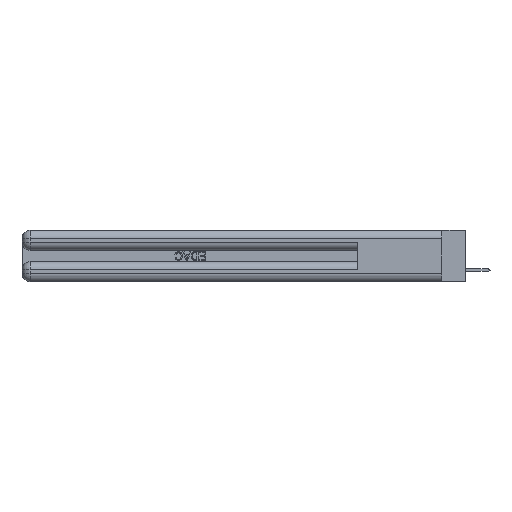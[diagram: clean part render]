
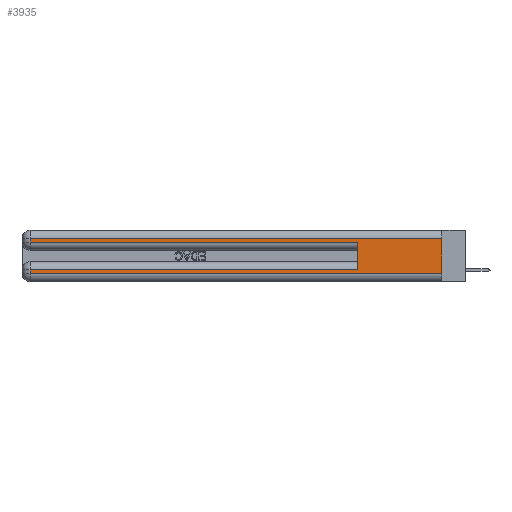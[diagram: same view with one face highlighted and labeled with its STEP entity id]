
A CAD part, left-side view. The second image highlights one B-rep face of the part: STEP entity #3935.
In plain terms, the highlighted planar face has unit normal (-1, 0, 0).
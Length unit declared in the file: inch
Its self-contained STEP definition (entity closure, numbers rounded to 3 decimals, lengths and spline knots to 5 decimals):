
#393 = ORIENTED_EDGE ( 'NONE', *, *, #5907, .F. ) ;
#418 = DIRECTION ( 'NONE',  ( 0., -1., 0. ) ) ;
#877 = VECTOR ( 'NONE', #418, 39.37008 ) ;
#1782 = ORIENTED_EDGE ( 'NONE', *, *, #13395, .T. ) ;
#3054 = DIRECTION ( 'NONE',  ( 0., 0., -1. ) ) ;
#3144 = EDGE_CURVE ( 'NONE', #14820, #27483, #23583, .T. ) ;
#3613 = VECTOR ( 'NONE', #27817, 39.37008 ) ;
#3715 = CARTESIAN_POINT ( 'NONE',  ( 0., 0., 0.31 ) ) ;
#3935 = ADVANCED_FACE ( 'NONE', ( #10803 ), #21529, .F. ) ;
#4452 = LINE ( 'NONE', #12826, #22128 ) ;
#4859 = CARTESIAN_POINT ( 'NONE',  ( 0., 0.6, 0.085 ) ) ;
#5136 = CARTESIAN_POINT ( 'NONE',  ( 0., 2.94, 0.37 ) ) ;
#5847 = EDGE_CURVE ( 'NONE', #24439, #14976, #4452, .T. ) ;
#5859 = LINE ( 'NONE', #25471, #12469 ) ;
#5907 = EDGE_CURVE ( 'NONE', #8286, #31642, #16191, .T. ) ;
#5970 = DIRECTION ( 'NONE',  ( 0., 1., 0. ) ) ;
#6474 = AXIS2_PLACEMENT_3D ( 'NONE', #27050, #18943, #21776 ) ;
#8118 = CARTESIAN_POINT ( 'NONE',  ( 0., 0., 0.085 ) ) ;
#8179 = EDGE_CURVE ( 'NONE', #27483, #14976, #20949, .T. ) ;
#8286 = VERTEX_POINT ( 'NONE', #3715 ) ;
#9301 = CARTESIAN_POINT ( 'NONE',  ( 0., 2.94, 0.06 ) ) ;
#10371 = EDGE_CURVE ( 'NONE', #8286, #14820, #5859, .T. ) ;
#10536 = VERTEX_POINT ( 'NONE', #9301 ) ;
#10803 = FACE_OUTER_BOUND ( 'NONE', #24010, .T. ) ;
#11311 = VECTOR ( 'NONE', #13959, 39.37008 ) ;
#11313 = VECTOR ( 'NONE', #19133, 39.37008 ) ;
#12422 = CARTESIAN_POINT ( 'NONE',  ( 0., 2.94, 0.285 ) ) ;
#12469 = VECTOR ( 'NONE', #5970, 39.37008 ) ;
#12826 = CARTESIAN_POINT ( 'NONE',  ( 0., 0.6, 0.145 ) ) ;
#13395 = EDGE_CURVE ( 'NONE', #15026, #10536, #22285, .T. ) ;
#13959 = DIRECTION ( 'NONE',  ( 0., 0., -1. ) ) ;
#14812 = ORIENTED_EDGE ( 'NONE', *, *, #29637, .T. ) ;
#14820 = VERTEX_POINT ( 'NONE', #27660 ) ;
#14976 = VERTEX_POINT ( 'NONE', #28220 ) ;
#15026 = VERTEX_POINT ( 'NONE', #27530 ) ;
#15793 = DIRECTION ( 'NONE',  ( 0., 0., 1. ) ) ;
#15957 = EDGE_CURVE ( 'NONE', #24439, #15026, #34412, .T. ) ;
#16191 = LINE ( 'NONE', #27192, #11311 ) ;
#18046 = ORIENTED_EDGE ( 'NONE', *, *, #5847, .F. ) ;
#18360 = CARTESIAN_POINT ( 'NONE',  ( 0., 0., 0.06 ) ) ;
#18943 = DIRECTION ( 'NONE',  ( 1., 0., 0. ) ) ;
#19133 = DIRECTION ( 'NONE',  ( 0., -1., 0. ) ) ;
#19674 = CARTESIAN_POINT ( 'NONE',  ( 0., 2.94, 0.37 ) ) ;
#20949 = LINE ( 'NONE', #30680, #11313 ) ;
#21529 = PLANE ( 'NONE',  #6474 ) ;
#21776 = DIRECTION ( 'NONE',  ( 0., 0., -1. ) ) ;
#22128 = VECTOR ( 'NONE', #15793, 39.37008 ) ;
#22285 = LINE ( 'NONE', #5136, #24926 ) ;
#23583 = LINE ( 'NONE', #19674, #35911 ) ;
#24010 = EDGE_LOOP ( 'NONE', ( #393, #34874, #29094, #24215, #18046, #29300, #1782, #14812 ) ) ;
#24215 = ORIENTED_EDGE ( 'NONE', *, *, #8179, .T. ) ;
#24439 = VERTEX_POINT ( 'NONE', #4859 ) ;
#24474 = DIRECTION ( 'NONE',  ( 0., 0., -1. ) ) ;
#24926 = VECTOR ( 'NONE', #24474, 39.37008 ) ;
#25471 = CARTESIAN_POINT ( 'NONE',  ( 0., 0., 0.31 ) ) ;
#27050 = CARTESIAN_POINT ( 'NONE',  ( 0., 0., 0.37 ) ) ;
#27192 = CARTESIAN_POINT ( 'NONE',  ( 0., 0., 0.37 ) ) ;
#27483 = VERTEX_POINT ( 'NONE', #12422 ) ;
#27530 = CARTESIAN_POINT ( 'NONE',  ( 0., 2.94, 0.085 ) ) ;
#27660 = CARTESIAN_POINT ( 'NONE',  ( 0., 2.94, 0.31 ) ) ;
#27817 = DIRECTION ( 'NONE',  ( 0., 1., 0. ) ) ;
#28220 = CARTESIAN_POINT ( 'NONE',  ( 0., 0.6, 0.285 ) ) ;
#29094 = ORIENTED_EDGE ( 'NONE', *, *, #3144, .T. ) ;
#29300 = ORIENTED_EDGE ( 'NONE', *, *, #15957, .T. ) ;
#29637 = EDGE_CURVE ( 'NONE', #10536, #31642, #35685, .T. ) ;
#30680 = CARTESIAN_POINT ( 'NONE',  ( 0., 0., 0.285 ) ) ;
#31642 = VERTEX_POINT ( 'NONE', #18360 ) ;
#33703 = CARTESIAN_POINT ( 'NONE',  ( 0., 0., 0.06 ) ) ;
#34412 = LINE ( 'NONE', #8118, #3613 ) ;
#34874 = ORIENTED_EDGE ( 'NONE', *, *, #10371, .T. ) ;
#35685 = LINE ( 'NONE', #33703, #877 ) ;
#35911 = VECTOR ( 'NONE', #3054, 39.37008 ) ;
